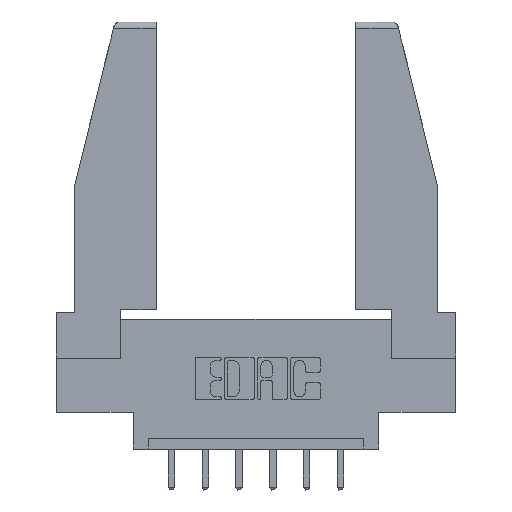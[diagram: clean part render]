
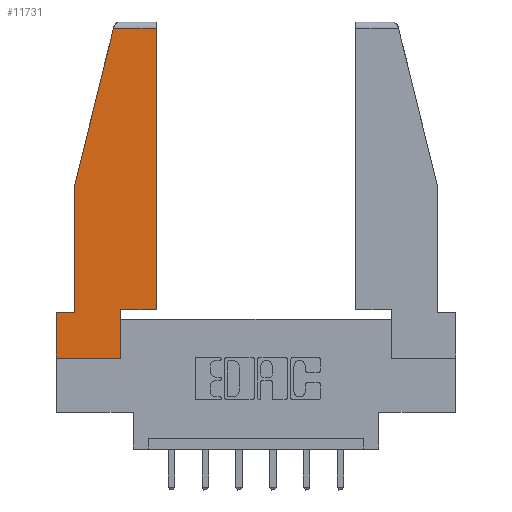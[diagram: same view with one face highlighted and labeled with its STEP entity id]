
A CAD part, top view. The second image highlights one B-rep face of the part: STEP entity #11731.
In plain terms, the highlighted planar face has unit normal (0, 0, 1).
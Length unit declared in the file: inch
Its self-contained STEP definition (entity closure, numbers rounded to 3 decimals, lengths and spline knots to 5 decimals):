
#271 = CARTESIAN_POINT ( 'NONE',  ( 0., 0.21, 0. ) ) ;
#880 = DIRECTION ( 'NONE',  ( -1., 0., 0. ) ) ;
#1111 = EDGE_CURVE ( 'NONE', #5402, #5617, #2642, .T. ) ;
#1231 = CARTESIAN_POINT ( 'NONE',  ( 0.086, 0.8, 0. ) ) ;
#1529 = DIRECTION ( 'NONE',  ( 1., 0., 0. ) ) ;
#1728 = VERTEX_POINT ( 'NONE', #10438 ) ;
#2188 = LINE ( 'NONE', #5556, #10592 ) ;
#2477 = VERTEX_POINT ( 'NONE', #271 ) ;
#2610 = CARTESIAN_POINT ( 'NONE',  ( 0.461, 0.223, 0. ) ) ;
#2642 = LINE ( 'NONE', #4250, #7823 ) ;
#2740 = CARTESIAN_POINT ( 'NONE',  ( 0.297, 0., 0. ) ) ;
#2763 = EDGE_CURVE ( 'NONE', #5617, #4524, #10999, .T. ) ;
#2812 = DIRECTION ( 'NONE',  ( -1., 0., 0. ) ) ;
#2815 = DIRECTION ( 'NONE',  ( -0.239, -0.971, 0. ) ) ;
#3262 = ORIENTED_EDGE ( 'NONE', *, *, #7507, .T. ) ;
#3284 = CARTESIAN_POINT ( 'NONE',  ( 0., 0., 0. ) ) ;
#3405 = EDGE_CURVE ( 'NONE', #1728, #2477, #9425, .T. ) ;
#3564 = EDGE_CURVE ( 'NONE', #9105, #5402, #7895, .T. ) ;
#3761 = CARTESIAN_POINT ( 'NONE',  ( 0.271, 1.55, 0. ) ) ;
#3854 = ORIENTED_EDGE ( 'NONE', *, *, #3405, .T. ) ;
#4178 = LINE ( 'NONE', #3284, #5180 ) ;
#4230 = DIRECTION ( 'NONE',  ( 1., 0., 0. ) ) ;
#4250 = CARTESIAN_POINT ( 'NONE',  ( 0.297, 0.223, 0. ) ) ;
#4361 = DIRECTION ( 'NONE',  ( 0., 0., 1. ) ) ;
#4524 = VERTEX_POINT ( 'NONE', #11376 ) ;
#4547 = ORIENTED_EDGE ( 'NONE', *, *, #5555, .T. ) ;
#4647 = ORIENTED_EDGE ( 'NONE', *, *, #10433, .T. ) ;
#4923 = LINE ( 'NONE', #11577, #7064 ) ;
#4963 = EDGE_CURVE ( 'NONE', #11702, #10405, #5679, .T. ) ;
#5180 = VECTOR ( 'NONE', #4230, 39.37008 ) ;
#5301 = PLANE ( 'NONE',  #8335 ) ;
#5402 = VERTEX_POINT ( 'NONE', #6371 ) ;
#5413 = EDGE_LOOP ( 'NONE', ( #6524, #4547, #6891, #4647, #3854, #3262, #11356, #7622, #5417 ) ) ;
#5417 = ORIENTED_EDGE ( 'NONE', *, *, #1111, .T. ) ;
#5445 = VECTOR ( 'NONE', #7819, 39.37008 ) ;
#5555 = EDGE_CURVE ( 'NONE', #4524, #11702, #2188, .T. ) ;
#5556 = CARTESIAN_POINT ( 'NONE',  ( 0., 1.52, 0. ) ) ;
#5617 = VERTEX_POINT ( 'NONE', #8620 ) ;
#5629 = VERTEX_POINT ( 'NONE', #8668 ) ;
#5679 = LINE ( 'NONE', #3761, #10191 ) ;
#6371 = CARTESIAN_POINT ( 'NONE',  ( 0.297, 0.223, 0. ) ) ;
#6524 = ORIENTED_EDGE ( 'NONE', *, *, #2763, .T. ) ;
#6613 = LINE ( 'NONE', #1231, #5445 ) ;
#6632 = VECTOR ( 'NONE', #10035, 39.37008 ) ;
#6891 = ORIENTED_EDGE ( 'NONE', *, *, #4963, .T. ) ;
#7064 = VECTOR ( 'NONE', #8001, 39.37008 ) ;
#7196 = CARTESIAN_POINT ( 'NONE',  ( 0.2636, 1.52, 0. ) ) ;
#7445 = CARTESIAN_POINT ( 'NONE',  ( 0., 0.21, 0. ) ) ;
#7507 = EDGE_CURVE ( 'NONE', #2477, #5629, #4923, .T. ) ;
#7622 = ORIENTED_EDGE ( 'NONE', *, *, #3564, .T. ) ;
#7819 = DIRECTION ( 'NONE',  ( 0., -1., 0. ) ) ;
#7823 = VECTOR ( 'NONE', #1529, 39.37008 ) ;
#7895 = LINE ( 'NONE', #2740, #6632 ) ;
#7902 = EDGE_CURVE ( 'NONE', #5629, #9105, #4178, .T. ) ;
#7903 = VECTOR ( 'NONE', #2812, 39.37008 ) ;
#8001 = DIRECTION ( 'NONE',  ( 0., -1., 0. ) ) ;
#8043 = DIRECTION ( 'NONE',  ( 1., 0., 0. ) ) ;
#8335 = AXIS2_PLACEMENT_3D ( 'NONE', #9762, #4361, #8043 ) ;
#8594 = VECTOR ( 'NONE', #9042, 39.37008 ) ;
#8620 = CARTESIAN_POINT ( 'NONE',  ( 0.461, 0.223, 0. ) ) ;
#8668 = CARTESIAN_POINT ( 'NONE',  ( 0., 0., 0. ) ) ;
#8981 = FACE_OUTER_BOUND ( 'NONE', #5413, .T. ) ;
#9042 = DIRECTION ( 'NONE',  ( 0., 1., 0. ) ) ;
#9105 = VERTEX_POINT ( 'NONE', #9493 ) ;
#9425 = LINE ( 'NONE', #7445, #7903 ) ;
#9493 = CARTESIAN_POINT ( 'NONE',  ( 0.297, 0., 0. ) ) ;
#9762 = CARTESIAN_POINT ( 'NONE',  ( 0., 0., 0. ) ) ;
#10035 = DIRECTION ( 'NONE',  ( 0., 1., 0. ) ) ;
#10191 = VECTOR ( 'NONE', #2815, 39.37008 ) ;
#10405 = VERTEX_POINT ( 'NONE', #11368 ) ;
#10433 = EDGE_CURVE ( 'NONE', #10405, #1728, #6613, .T. ) ;
#10438 = CARTESIAN_POINT ( 'NONE',  ( 0.086, 0.21, 0. ) ) ;
#10592 = VECTOR ( 'NONE', #880, 39.37008 ) ;
#10999 = LINE ( 'NONE', #2610, #8594 ) ;
#11356 = ORIENTED_EDGE ( 'NONE', *, *, #7902, .T. ) ;
#11368 = CARTESIAN_POINT ( 'NONE',  ( 0.086, 0.8, 0. ) ) ;
#11376 = CARTESIAN_POINT ( 'NONE',  ( 0.461, 1.52, 0. ) ) ;
#11577 = CARTESIAN_POINT ( 'NONE',  ( 0., 0.21, 0. ) ) ;
#11702 = VERTEX_POINT ( 'NONE', #7196 ) ;
#11731 = ADVANCED_FACE ( 'NONE', ( #8981 ), #5301, .T. ) ;
